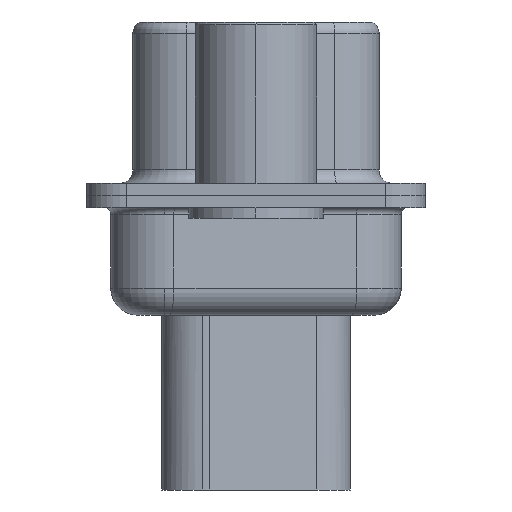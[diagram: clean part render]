
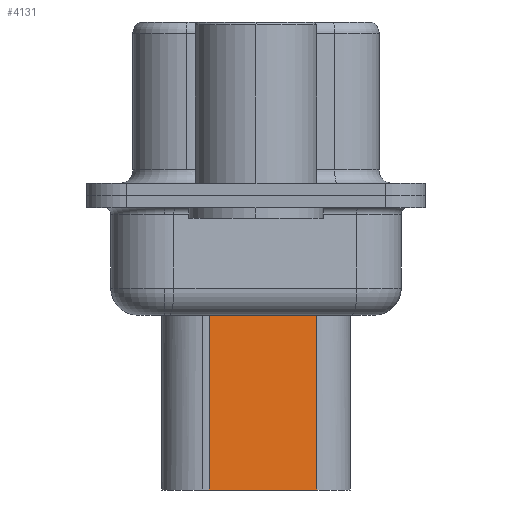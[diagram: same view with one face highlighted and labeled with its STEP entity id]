
A CAD part, left-side view. The second image highlights one B-rep face of the part: STEP entity #4131.
In plain terms, the highlighted planar face has unit normal (-0.985, -0.174, 0).
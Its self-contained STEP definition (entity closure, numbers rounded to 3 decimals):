
#125 = DIRECTION ( 'NONE',  ( 0., 0., -1. ) ) ;
#400 = EDGE_CURVE ( 'NONE', #4570, #12456, #4696, .T. ) ;
#904 = ORIENTED_EDGE ( 'NONE', *, *, #2337, .F. ) ;
#1478 = DIRECTION ( 'NONE',  ( 0., 0., -1. ) ) ;
#1786 = VECTOR ( 'NONE', #8209, 1000. ) ;
#2131 = DIRECTION ( 'NONE',  ( 0.174, -0.985, 0. ) ) ;
#2337 = EDGE_CURVE ( 'NONE', #9948, #5320, #15505, .T. ) ;
#2358 = CARTESIAN_POINT ( 'NONE',  ( 4.524, 1.74, -10.95 ) ) ;
#2466 = AXIS2_PLACEMENT_3D ( 'NONE', #14893, #14988, #2131 ) ;
#2915 = LINE ( 'NONE', #5981, #14536 ) ;
#4131 = ADVANCED_FACE ( 'NONE', ( #10464 ), #15275, .T. ) ;
#4177 = CARTESIAN_POINT ( 'NONE',  ( 5.229, -2.26, -3.1 ) ) ;
#4570 = VERTEX_POINT ( 'NONE', #12258 ) ;
#4696 = LINE ( 'NONE', #9195, #5216 ) ;
#4777 = VECTOR ( 'NONE', #125, 1000. ) ;
#5216 = VECTOR ( 'NONE', #10837, 1000. ) ;
#5320 = VERTEX_POINT ( 'NONE', #17044 ) ;
#5981 = CARTESIAN_POINT ( 'NONE',  ( 4.524, 1.74, -3.1 ) ) ;
#8209 = DIRECTION ( 'NONE',  ( -0.174, 0.985, 0. ) ) ;
#9195 = CARTESIAN_POINT ( 'NONE',  ( 4.353, 2.709, -3.975 ) ) ;
#9510 = ORIENTED_EDGE ( 'NONE', *, *, #16694, .F. ) ;
#9948 = VERTEX_POINT ( 'NONE', #18663 ) ;
#10464 = FACE_OUTER_BOUND ( 'NONE', #15492, .T. ) ;
#10837 = DIRECTION ( 'NONE',  ( -0.174, 0.985, 0. ) ) ;
#12258 = CARTESIAN_POINT ( 'NONE',  ( 5.229, -2.26, -3.975 ) ) ;
#12456 = VERTEX_POINT ( 'NONE', #13769 ) ;
#13066 = ORIENTED_EDGE ( 'NONE', *, *, #15116, .T. ) ;
#13769 = CARTESIAN_POINT ( 'NONE',  ( 4.524, 1.74, -3.975 ) ) ;
#14536 = VECTOR ( 'NONE', #1478, 1000. ) ;
#14893 = CARTESIAN_POINT ( 'NONE',  ( 4.524, 1.74, -3.1 ) ) ;
#14988 = DIRECTION ( 'NONE',  ( -0.985, -0.174, 0. ) ) ;
#15116 = EDGE_CURVE ( 'NONE', #12456, #5320, #2915, .T. ) ;
#15275 = PLANE ( 'NONE',  #2466 ) ;
#15492 = EDGE_LOOP ( 'NONE', ( #9510, #16036, #13066, #904 ) ) ;
#15505 = LINE ( 'NONE', #2358, #1786 ) ;
#16036 = ORIENTED_EDGE ( 'NONE', *, *, #400, .T. ) ;
#16694 = EDGE_CURVE ( 'NONE', #4570, #9948, #17339, .T. ) ;
#17044 = CARTESIAN_POINT ( 'NONE',  ( 4.524, 1.74, -10.95 ) ) ;
#17339 = LINE ( 'NONE', #4177, #4777 ) ;
#18663 = CARTESIAN_POINT ( 'NONE',  ( 5.229, -2.26, -10.95 ) ) ;
